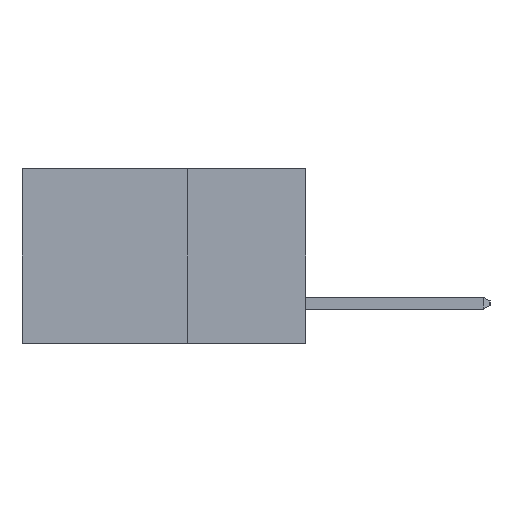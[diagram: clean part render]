
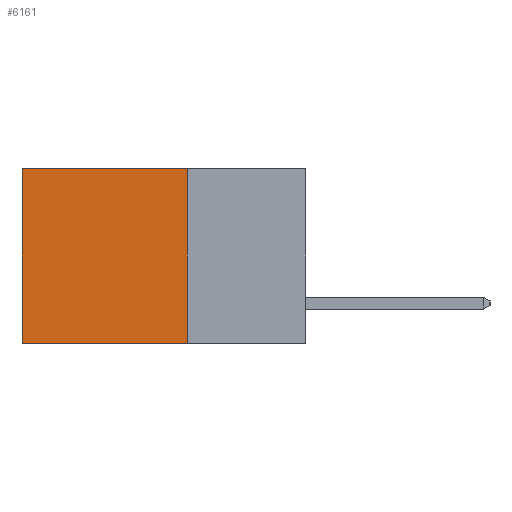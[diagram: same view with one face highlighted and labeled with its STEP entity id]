
A CAD part, left-side view. The second image highlights one B-rep face of the part: STEP entity #6161.
In plain terms, the highlighted planar face has unit normal (-1, 0, 0).
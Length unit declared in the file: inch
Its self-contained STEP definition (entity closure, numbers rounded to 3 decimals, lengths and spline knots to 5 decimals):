
#481 = EDGE_CURVE ( 'NONE', #16660, #24731, #25459, .T. ) ;
#907 = ORIENTED_EDGE ( 'NONE', *, *, #13789, .F. ) ;
#3081 = DIRECTION ( 'NONE',  ( 0., 0., -1. ) ) ;
#3168 = DIRECTION ( 'NONE',  ( 1., 0., 0. ) ) ;
#3171 = CARTESIAN_POINT ( 'NONE',  ( 0.298, 0.25, 0. ) ) ;
#3259 = LINE ( 'NONE', #13313, #13858 ) ;
#3321 = PLANE ( 'NONE',  #22249 ) ;
#3362 = EDGE_CURVE ( 'NONE', #3671, #17904, #19163, .T. ) ;
#3671 = VERTEX_POINT ( 'NONE', #22596 ) ;
#6161 = ADVANCED_FACE ( 'NONE', ( #17333 ), #3321, .F. ) ;
#6462 = DIRECTION ( 'NONE',  ( 0., 0., -1. ) ) ;
#6818 = CARTESIAN_POINT ( 'NONE',  ( 0.298, 0.6, 0. ) ) ;
#7015 = CARTESIAN_POINT ( 'NONE',  ( 0.298, 0.25, 0. ) ) ;
#7091 = CARTESIAN_POINT ( 'NONE',  ( 0.298, 0.25, -0.37 ) ) ;
#8620 = EDGE_CURVE ( 'NONE', #17904, #24731, #20866, .T. ) ;
#8716 = DIRECTION ( 'NONE',  ( 0., 1., 0. ) ) ;
#9131 = ORIENTED_EDGE ( 'NONE', *, *, #481, .F. ) ;
#9814 = VECTOR ( 'NONE', #6462, 39.37008 ) ;
#11216 = CARTESIAN_POINT ( 'NONE',  ( 0.298, 0.6, 0. ) ) ;
#13245 = ORIENTED_EDGE ( 'NONE', *, *, #3362, .T. ) ;
#13313 = CARTESIAN_POINT ( 'NONE',  ( 0.298, 0.25, 0. ) ) ;
#13789 = EDGE_CURVE ( 'NONE', #3671, #16660, #3259, .T. ) ;
#13858 = VECTOR ( 'NONE', #23090, 39.37008 ) ;
#15708 = EDGE_LOOP ( 'NONE', ( #21371, #9131, #907, #13245 ) ) ;
#16660 = VERTEX_POINT ( 'NONE', #7091 ) ;
#17141 = CARTESIAN_POINT ( 'NONE',  ( 0.298, 0.6, -0.37 ) ) ;
#17333 = FACE_OUTER_BOUND ( 'NONE', #15708, .T. ) ;
#17904 = VERTEX_POINT ( 'NONE', #11216 ) ;
#18559 = VECTOR ( 'NONE', #8716, 39.37008 ) ;
#19163 = LINE ( 'NONE', #7015, #18559 ) ;
#20866 = LINE ( 'NONE', #6818, #9814 ) ;
#20914 = CARTESIAN_POINT ( 'NONE',  ( 0.298, 0.25, -0.37 ) ) ;
#21371 = ORIENTED_EDGE ( 'NONE', *, *, #8620, .T. ) ;
#22249 = AXIS2_PLACEMENT_3D ( 'NONE', #3171, #3168, #3081 ) ;
#22596 = CARTESIAN_POINT ( 'NONE',  ( 0.298, 0.25, 0. ) ) ;
#23090 = DIRECTION ( 'NONE',  ( 0., 0., -1. ) ) ;
#24731 = VERTEX_POINT ( 'NONE', #17141 ) ;
#24843 = VECTOR ( 'NONE', #25300, 39.37008 ) ;
#25300 = DIRECTION ( 'NONE',  ( 0., 1., 0. ) ) ;
#25459 = LINE ( 'NONE', #20914, #24843 ) ;
